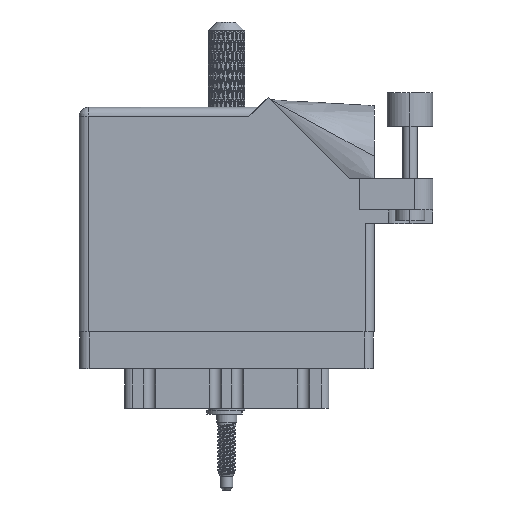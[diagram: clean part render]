
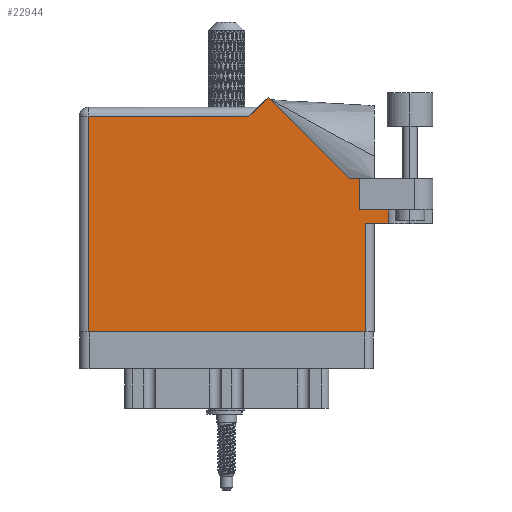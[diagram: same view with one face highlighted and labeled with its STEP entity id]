
A CAD part, front view. The second image highlights one B-rep face of the part: STEP entity #22944.
In plain terms, the highlighted face is planar.
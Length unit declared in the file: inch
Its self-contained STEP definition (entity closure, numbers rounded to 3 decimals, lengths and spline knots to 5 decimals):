
#1680 = LINE ( 'NONE', #81398, #41370 ) ;
#4038 = LINE ( 'NONE', #41336, #96114 ) ;
#6161 = FACE_OUTER_BOUND ( 'NONE', #45914, .T. ) ;
#6651 = LINE ( 'NONE', #99625, #10287 ) ;
#7845 = CARTESIAN_POINT ( 'NONE',  ( 1.217, 1.53, 0. ) ) ;
#8183 = EDGE_CURVE ( 'NONE', #9064, #93389, #17741, .T. ) ;
#8634 = VERTEX_POINT ( 'NONE', #30321 ) ;
#8950 = ORIENTED_EDGE ( 'NONE', *, *, #81021, .T. ) ;
#9064 = VERTEX_POINT ( 'NONE', #88962 ) ;
#10161 = EDGE_CURVE ( 'NONE', #22237, #32851, #4038, .T. ) ;
#10287 = VECTOR ( 'NONE', #60319, 39.37008 ) ;
#10853 = ORIENTED_EDGE ( 'NONE', *, *, #99104, .T. ) ;
#12834 = LINE ( 'NONE', #34342, #24843 ) ;
#17741 = LINE ( 'NONE', #80123, #57066 ) ;
#21873 = EDGE_CURVE ( 'NONE', #48996, #52620, #1680, .T. ) ;
#22237 = VERTEX_POINT ( 'NONE', #53501 ) ;
#22481 = CARTESIAN_POINT ( 'NONE',  ( 0., 1.53, 0. ) ) ;
#22944 = ADVANCED_FACE ( 'NONE', ( #6161 ), #100143, .F. ) ;
#24281 = CARTESIAN_POINT ( 'NONE',  ( 1.948, 0., 0. ) ) ;
#24843 = VECTOR ( 'NONE', #96678, 39.37008 ) ;
#24917 = CARTESIAN_POINT ( 'NONE',  ( 2.1115, 1.16177, 0. ) ) ;
#30321 = CARTESIAN_POINT ( 'NONE',  ( 1.28771, 1.60071, 0. ) ) ;
#32843 = CARTESIAN_POINT ( 'NONE',  ( 1.84442, 1.044, 0. ) ) ;
#32847 = DIRECTION ( 'NONE',  ( 1., 0., 0. ) ) ;
#32851 = VERTEX_POINT ( 'NONE', #24281 ) ;
#34342 = CARTESIAN_POINT ( 'NONE',  ( 0., 1.468, 0. ) ) ;
#34792 = DIRECTION ( 'NONE',  ( 0., 1., 0. ) ) ;
#38874 = ORIENTED_EDGE ( 'NONE', *, *, #66129, .F. ) ;
#39004 = LINE ( 'NONE', #7845, #47537 ) ;
#39491 = CARTESIAN_POINT ( 'NONE',  ( 1.948, 0.737, 0. ) ) ;
#40085 = CARTESIAN_POINT ( 'NONE',  ( 1.91, 1.044, 0. ) ) ;
#41336 = CARTESIAN_POINT ( 'NONE',  ( 0., 0., 0. ) ) ;
#41370 = VECTOR ( 'NONE', #32847, 39.37008 ) ;
#43363 = EDGE_CURVE ( 'NONE', #48996, #93000, #57795, .T. ) ;
#43473 = ORIENTED_EDGE ( 'NONE', *, *, #10161, .T. ) ;
#44366 = ORIENTED_EDGE ( 'NONE', *, *, #66133, .T. ) ;
#45914 = EDGE_LOOP ( 'NONE', ( #43473, #93968, #50182, #38874, #100407, #71745, #60217, #92623, #8950, #10853, #44366 ) ) ;
#47537 = VECTOR ( 'NONE', #71691, 39.37008 ) ;
#48440 = CARTESIAN_POINT ( 'NONE',  ( 0.062, 0., 0. ) ) ;
#48996 = VERTEX_POINT ( 'NONE', #58640 ) ;
#49145 = VECTOR ( 'NONE', #34792, 39.37008 ) ;
#49470 = VECTOR ( 'NONE', #83702, 39.37008 ) ;
#50045 = DIRECTION ( 'NONE',  ( 1., 0., 0. ) ) ;
#50182 = ORIENTED_EDGE ( 'NONE', *, *, #8183, .T. ) ;
#52337 = VECTOR ( 'NONE', #80133, 39.37008 ) ;
#52620 = VERTEX_POINT ( 'NONE', #56785 ) ;
#53455 = EDGE_CURVE ( 'NONE', #93000, #81019, #6651, .T. ) ;
#53501 = CARTESIAN_POINT ( 'NONE',  ( 0.062, 0., 0. ) ) ;
#55611 = VECTOR ( 'NONE', #79623, 39.37008 ) ;
#56110 = LINE ( 'NONE', #48440, #55611 ) ;
#56785 = CARTESIAN_POINT ( 'NONE',  ( 2.1115, 0.831, 0. ) ) ;
#57066 = VECTOR ( 'NONE', #78096, 39.37008 ) ;
#57795 = LINE ( 'NONE', #73630, #49145 ) ;
#58207 = CARTESIAN_POINT ( 'NONE',  ( 1.84442, 1.044, 0. ) ) ;
#58640 = CARTESIAN_POINT ( 'NONE',  ( 1.91, 0.831, 0. ) ) ;
#60217 = ORIENTED_EDGE ( 'NONE', *, *, #53455, .T. ) ;
#60319 = DIRECTION ( 'NONE',  ( -1., 0., 0. ) ) ;
#62989 = CARTESIAN_POINT ( 'NONE',  ( 2.1115, 0.737, 0. ) ) ;
#63036 = VERTEX_POINT ( 'NONE', #86342 ) ;
#66129 = EDGE_CURVE ( 'NONE', #52620, #93389, #78610, .T. ) ;
#66133 = EDGE_CURVE ( 'NONE', #63036, #22237, #56110, .T. ) ;
#67495 = DIRECTION ( 'NONE',  ( -1., 0., 0. ) ) ;
#71691 = DIRECTION ( 'NONE',  ( -0.707, -0.707, 0. ) ) ;
#71745 = ORIENTED_EDGE ( 'NONE', *, *, #43363, .T. ) ;
#72342 = CARTESIAN_POINT ( 'NONE',  ( 1.155, 1.468, 0. ) ) ;
#73630 = CARTESIAN_POINT ( 'NONE',  ( 1.91, 0.831, 0. ) ) ;
#75536 = LINE ( 'NONE', #58207, #49470 ) ;
#76182 = DIRECTION ( 'NONE',  ( 0., 0., -1. ) ) ;
#77841 = VERTEX_POINT ( 'NONE', #72342 ) ;
#78096 = DIRECTION ( 'NONE',  ( 1., 0., 0. ) ) ;
#78350 = LINE ( 'NONE', #39491, #96651 ) ;
#78610 = LINE ( 'NONE', #24917, #52337 ) ;
#78893 = AXIS2_PLACEMENT_3D ( 'NONE', #22481, #76182, #67495 ) ;
#79623 = DIRECTION ( 'NONE',  ( 0., -1., 0. ) ) ;
#79984 = EDGE_CURVE ( 'NONE', #32851, #9064, #78350, .T. ) ;
#80123 = CARTESIAN_POINT ( 'NONE',  ( 2.01, 0.737, 0. ) ) ;
#80133 = DIRECTION ( 'NONE',  ( 0., -1., 0. ) ) ;
#81019 = VERTEX_POINT ( 'NONE', #32843 ) ;
#81021 = EDGE_CURVE ( 'NONE', #8634, #77841, #39004, .T. ) ;
#81398 = CARTESIAN_POINT ( 'NONE',  ( 1.91, 0.831, 0. ) ) ;
#83702 = DIRECTION ( 'NONE',  ( -0.707, 0.707, 0. ) ) ;
#86342 = CARTESIAN_POINT ( 'NONE',  ( 0.062, 1.468, 0. ) ) ;
#88962 = CARTESIAN_POINT ( 'NONE',  ( 1.948, 0.737, 0. ) ) ;
#92623 = ORIENTED_EDGE ( 'NONE', *, *, #96876, .T. ) ;
#93000 = VERTEX_POINT ( 'NONE', #40085 ) ;
#93389 = VERTEX_POINT ( 'NONE', #62989 ) ;
#93968 = ORIENTED_EDGE ( 'NONE', *, *, #79984, .T. ) ;
#94169 = DIRECTION ( 'NONE',  ( 0., 1., 0. ) ) ;
#96114 = VECTOR ( 'NONE', #50045, 39.37008 ) ;
#96651 = VECTOR ( 'NONE', #94169, 39.37008 ) ;
#96678 = DIRECTION ( 'NONE',  ( -1., 0., 0. ) ) ;
#96876 = EDGE_CURVE ( 'NONE', #81019, #8634, #75536, .T. ) ;
#99104 = EDGE_CURVE ( 'NONE', #77841, #63036, #12834, .T. ) ;
#99625 = CARTESIAN_POINT ( 'NONE',  ( 2.41, 1.044, 0. ) ) ;
#100143 = PLANE ( 'NONE',  #78893 ) ;
#100407 = ORIENTED_EDGE ( 'NONE', *, *, #21873, .F. ) ;
